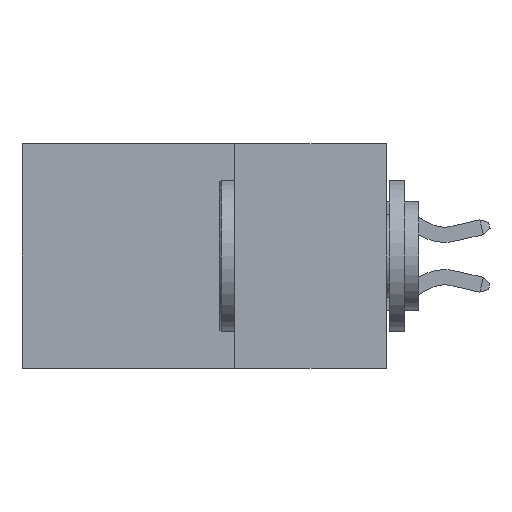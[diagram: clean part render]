
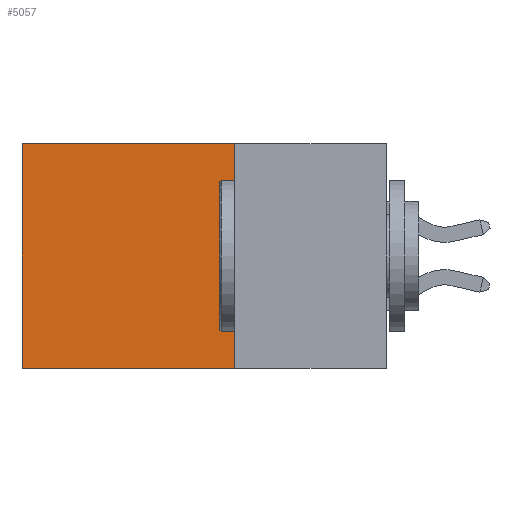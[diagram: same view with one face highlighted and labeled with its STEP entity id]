
A CAD part, left-side view. The second image highlights one B-rep face of the part: STEP entity #5057.
In plain terms, the highlighted planar face has unit normal (-1, 0, 0).
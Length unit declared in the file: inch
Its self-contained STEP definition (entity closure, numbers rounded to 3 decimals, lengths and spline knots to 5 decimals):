
#232 = CARTESIAN_POINT ( 'NONE',  ( 0.298, 0.25, 0. ) ) ;
#576 = FACE_OUTER_BOUND ( 'NONE', #6180, .T. ) ;
#1148 = LINE ( 'NONE', #12456, #7956 ) ;
#2060 = DIRECTION ( 'NONE',  ( 0., 1., 0. ) ) ;
#2220 = ORIENTED_EDGE ( 'NONE', *, *, #12393, .T. ) ;
#2628 = DIRECTION ( 'NONE',  ( 0., 0., -1. ) ) ;
#2663 = DIRECTION ( 'NONE',  ( 1., 0., 0. ) ) ;
#2692 = CARTESIAN_POINT ( 'NONE',  ( 0.298, 0.25, 0. ) ) ;
#2883 = PLANE ( 'NONE',  #18538 ) ;
#3753 = DIRECTION ( 'NONE',  ( 0., 0., -1. ) ) ;
#4190 = ORIENTED_EDGE ( 'NONE', *, *, #32457, .F. ) ;
#5057 = ADVANCED_FACE ( 'NONE', ( #576 ), #2883, .F. ) ;
#5531 = VECTOR ( 'NONE', #3753, 39.37008 ) ;
#6180 = EDGE_LOOP ( 'NONE', ( #2220, #16083, #4190, #19592 ) ) ;
#6594 = VERTEX_POINT ( 'NONE', #8973 ) ;
#7343 = DIRECTION ( 'NONE',  ( 0., 1., 0. ) ) ;
#7956 = VECTOR ( 'NONE', #7343, 39.37008 ) ;
#8973 = CARTESIAN_POINT ( 'NONE',  ( 0.298, 0.6, -0.37 ) ) ;
#9579 = EDGE_CURVE ( 'NONE', #22892, #6594, #1148, .T. ) ;
#9720 = LINE ( 'NONE', #26712, #29965 ) ;
#11527 = LINE ( 'NONE', #26645, #5531 ) ;
#12332 = LINE ( 'NONE', #19991, #19206 ) ;
#12393 = EDGE_CURVE ( 'NONE', #28364, #6594, #9720, .T. ) ;
#12456 = CARTESIAN_POINT ( 'NONE',  ( 0.298, 0.25, -0.37 ) ) ;
#16083 = ORIENTED_EDGE ( 'NONE', *, *, #9579, .F. ) ;
#18538 = AXIS2_PLACEMENT_3D ( 'NONE', #2692, #2663, #2628 ) ;
#19158 = DIRECTION ( 'NONE',  ( 0., 0., -1. ) ) ;
#19206 = VECTOR ( 'NONE', #2060, 39.37008 ) ;
#19517 = EDGE_CURVE ( 'NONE', #21475, #28364, #12332, .T. ) ;
#19592 = ORIENTED_EDGE ( 'NONE', *, *, #19517, .T. ) ;
#19991 = CARTESIAN_POINT ( 'NONE',  ( 0.298, 0.25, 0. ) ) ;
#21475 = VERTEX_POINT ( 'NONE', #232 ) ;
#22892 = VERTEX_POINT ( 'NONE', #23900 ) ;
#23900 = CARTESIAN_POINT ( 'NONE',  ( 0.298, 0.25, -0.37 ) ) ;
#24829 = CARTESIAN_POINT ( 'NONE',  ( 0.298, 0.6, 0. ) ) ;
#26645 = CARTESIAN_POINT ( 'NONE',  ( 0.298, 0.25, 0. ) ) ;
#26712 = CARTESIAN_POINT ( 'NONE',  ( 0.298, 0.6, 0. ) ) ;
#28364 = VERTEX_POINT ( 'NONE', #24829 ) ;
#29965 = VECTOR ( 'NONE', #19158, 39.37008 ) ;
#32457 = EDGE_CURVE ( 'NONE', #21475, #22892, #11527, .T. ) ;
